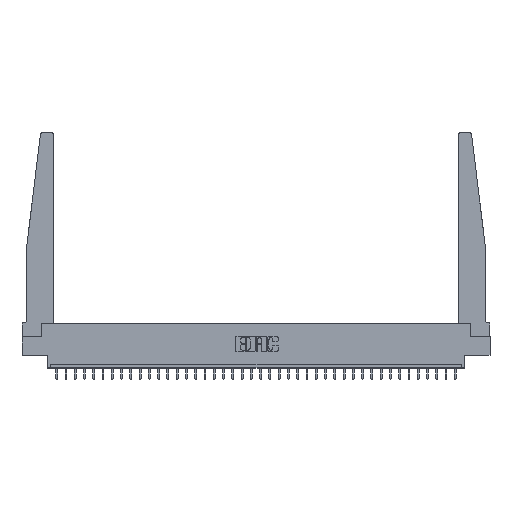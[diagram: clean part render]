
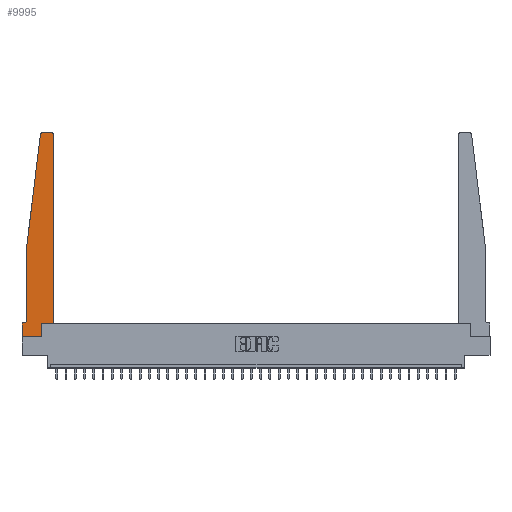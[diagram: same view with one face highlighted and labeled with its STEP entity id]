
A CAD part, top view. The second image highlights one B-rep face of the part: STEP entity #9995.
In plain terms, the highlighted planar face has unit normal (0, 0, 1).
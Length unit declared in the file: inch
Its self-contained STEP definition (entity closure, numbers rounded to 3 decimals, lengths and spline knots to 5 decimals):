
#300 = VERTEX_POINT ( 'NONE', #10481 ) ;
#734 = LINE ( 'NONE', #8101, #11076 ) ;
#1707 = DIRECTION ( 'NONE',  ( -0.122, -0.992, 0. ) ) ;
#1831 = FACE_OUTER_BOUND ( 'NONE', #9737, .T. ) ;
#2139 = EDGE_CURVE ( 'NONE', #7560, #2430, #734, .T. ) ;
#2144 = CARTESIAN_POINT ( 'NONE',  ( 0., 0., 0.37 ) ) ;
#2316 = CARTESIAN_POINT ( 'NONE',  ( 0.24675, 2.72367, 0.37 ) ) ;
#2386 = LINE ( 'NONE', #19761, #15559 ) ;
#2430 = VERTEX_POINT ( 'NONE', #7080 ) ;
#2535 = DIRECTION ( 'NONE',  ( 0., 0., -1. ) ) ;
#2603 = CARTESIAN_POINT ( 'NONE',  ( 0.425, 0.18, 0.37 ) ) ;
#2870 = DIRECTION ( 'NONE',  ( -1., 0., 0. ) ) ;
#3364 = DIRECTION ( 'NONE',  ( 0., -1., 0. ) ) ;
#3448 = AXIS2_PLACEMENT_3D ( 'NONE', #6725, #11809, #6570 ) ;
#3681 = EDGE_CURVE ( 'NONE', #2430, #6125, #12863, .T. ) ;
#4081 = CARTESIAN_POINT ( 'NONE',  ( 0.395, 2.75, 0.37 ) ) ;
#4702 = ORIENTED_EDGE ( 'NONE', *, *, #5469, .T. ) ;
#5469 = EDGE_CURVE ( 'NONE', #6577, #11866, #28727, .T. ) ;
#6125 = VERTEX_POINT ( 'NONE', #2316 ) ;
#6570 = DIRECTION ( 'NONE',  ( 1., 0., 0. ) ) ;
#6577 = VERTEX_POINT ( 'NONE', #20592 ) ;
#6643 = CARTESIAN_POINT ( 'NONE',  ( 0.2605, 0., 0.37 ) ) ;
#6725 = CARTESIAN_POINT ( 'NONE',  ( 0., 0.1875, 0.37 ) ) ;
#7080 = CARTESIAN_POINT ( 'NONE',  ( 0.27653, 2.75, 0.37 ) ) ;
#7560 = VERTEX_POINT ( 'NONE', #4081 ) ;
#7802 = EDGE_CURVE ( 'NONE', #300, #32115, #15045, .T. ) ;
#7805 = EDGE_CURVE ( 'NONE', #9225, #23556, #9787, .T. ) ;
#8101 = CARTESIAN_POINT ( 'NONE',  ( 0.25, 2.75, 0.37 ) ) ;
#9005 = DIRECTION ( 'NONE',  ( 1., 0., 0. ) ) ;
#9020 = CARTESIAN_POINT ( 'NONE',  ( 0., 0., 0.37 ) ) ;
#9225 = VERTEX_POINT ( 'NONE', #6643 ) ;
#9737 = EDGE_LOOP ( 'NONE', ( #20109, #15426, #15410, #4702, #16106, #26587, #24130, #14620, #29004, #9739, #24128, #9756 ) ) ;
#9739 = ORIENTED_EDGE ( 'NONE', *, *, #21697, .T. ) ;
#9756 = ORIENTED_EDGE ( 'NONE', *, *, #17944, .T. ) ;
#9787 = LINE ( 'NONE', #12593, #22171 ) ;
#9995 = ADVANCED_FACE ( 'NONE', ( #1831 ), #29013, .T. ) ;
#10481 = CARTESIAN_POINT ( 'NONE',  ( 0.425, 0.18, 0.37 ) ) ;
#10657 = DIRECTION ( 'NONE',  ( 1., 0., 0. ) ) ;
#10782 = LINE ( 'NONE', #21133, #31820 ) ;
#10863 = CARTESIAN_POINT ( 'NONE',  ( 0.065, 1.25, 0.37 ) ) ;
#10869 = AXIS2_PLACEMENT_3D ( 'NONE', #29723, #2535, #22856 ) ;
#11076 = VECTOR ( 'NONE', #2870, 39.37008 ) ;
#11333 = AXIS2_PLACEMENT_3D ( 'NONE', #21490, #31466, #9005 ) ;
#11809 = DIRECTION ( 'NONE',  ( 0., 0., 1. ) ) ;
#11866 = VERTEX_POINT ( 'NONE', #29800 ) ;
#12130 = DIRECTION ( 'NONE',  ( 0., -1., 0. ) ) ;
#12593 = CARTESIAN_POINT ( 'NONE',  ( 0.2605, 0.18, 0.37 ) ) ;
#12863 = CIRCLE ( 'NONE', #14942, 0.03 ) ;
#13383 = CARTESIAN_POINT ( 'NONE',  ( 0., 0., 0.37 ) ) ;
#14620 = ORIENTED_EDGE ( 'NONE', *, *, #26352, .T. ) ;
#14762 = VERTEX_POINT ( 'NONE', #32381 ) ;
#14942 = AXIS2_PLACEMENT_3D ( 'NONE', #15763, #18395, #10657 ) ;
#15045 = LINE ( 'NONE', #2603, #20067 ) ;
#15410 = ORIENTED_EDGE ( 'NONE', *, *, #22152, .T. ) ;
#15426 = ORIENTED_EDGE ( 'NONE', *, *, #3681, .T. ) ;
#15559 = VECTOR ( 'NONE', #16813, 39.37008 ) ;
#15763 = CARTESIAN_POINT ( 'NONE',  ( 0.27653, 2.72, 0.37 ) ) ;
#16106 = ORIENTED_EDGE ( 'NONE', *, *, #29680, .T. ) ;
#16571 = LINE ( 'NONE', #9020, #17307 ) ;
#16813 = DIRECTION ( 'NONE',  ( -1., 0., 0. ) ) ;
#17307 = VECTOR ( 'NONE', #24117, 39.37008 ) ;
#17919 = CARTESIAN_POINT ( 'NONE',  ( 0., 0.1875, 0.37 ) ) ;
#17944 = EDGE_CURVE ( 'NONE', #32115, #7560, #25486, .T. ) ;
#18082 = EDGE_CURVE ( 'NONE', #26295, #18791, #24584, .T. ) ;
#18395 = DIRECTION ( 'NONE',  ( 0., 0., 1. ) ) ;
#18791 = VERTEX_POINT ( 'NONE', #13383 ) ;
#18826 = DIRECTION ( 'NONE',  ( 1., 0., 0. ) ) ;
#19761 = CARTESIAN_POINT ( 'NONE',  ( 0.065, 0.1875, 0.37 ) ) ;
#20067 = VECTOR ( 'NONE', #32259, 39.37008 ) ;
#20109 = ORIENTED_EDGE ( 'NONE', *, *, #2139, .T. ) ;
#20200 = EDGE_CURVE ( 'NONE', #14762, #26295, #2386, .T. ) ;
#20592 = CARTESIAN_POINT ( 'NONE',  ( 0.065, 1.25, 0.37 ) ) ;
#21133 = CARTESIAN_POINT ( 'NONE',  ( 0.425, 0.18, 0.37 ) ) ;
#21490 = CARTESIAN_POINT ( 'NONE',  ( 0.395, 2.72, 0.37 ) ) ;
#21695 = CARTESIAN_POINT ( 'NONE',  ( 0.065, 1.25, 0.37 ) ) ;
#21697 = EDGE_CURVE ( 'NONE', #23556, #300, #10782, .T. ) ;
#21888 = CARTESIAN_POINT ( 'NONE',  ( 0.425, 2.72, 0.37 ) ) ;
#22152 = EDGE_CURVE ( 'NONE', #6125, #6577, #29214, .T. ) ;
#22171 = VECTOR ( 'NONE', #22602, 39.37008 ) ;
#22438 = VECTOR ( 'NONE', #1707, 39.37008 ) ;
#22602 = DIRECTION ( 'NONE',  ( 0., 1., 0. ) ) ;
#22856 = DIRECTION ( 'NONE',  ( -1., 0., 0. ) ) ;
#23556 = VERTEX_POINT ( 'NONE', #24685 ) ;
#24117 = DIRECTION ( 'NONE',  ( 1., 0., 0. ) ) ;
#24128 = ORIENTED_EDGE ( 'NONE', *, *, #7802, .T. ) ;
#24130 = ORIENTED_EDGE ( 'NONE', *, *, #18082, .T. ) ;
#24584 = LINE ( 'NONE', #2144, #29656 ) ;
#24685 = CARTESIAN_POINT ( 'NONE',  ( 0.2605, 0.18, 0.37 ) ) ;
#25486 = CIRCLE ( 'NONE', #11333, 0.03 ) ;
#25551 = CIRCLE ( 'NONE', #10869, 0.05 ) ;
#26295 = VERTEX_POINT ( 'NONE', #17919 ) ;
#26352 = EDGE_CURVE ( 'NONE', #18791, #9225, #16571, .T. ) ;
#26587 = ORIENTED_EDGE ( 'NONE', *, *, #20200, .T. ) ;
#28727 = LINE ( 'NONE', #10863, #29702 ) ;
#29004 = ORIENTED_EDGE ( 'NONE', *, *, #7805, .T. ) ;
#29013 = PLANE ( 'NONE',  #3448 ) ;
#29214 = LINE ( 'NONE', #21695, #22438 ) ;
#29656 = VECTOR ( 'NONE', #12130, 39.37008 ) ;
#29680 = EDGE_CURVE ( 'NONE', #11866, #14762, #25551, .T. ) ;
#29702 = VECTOR ( 'NONE', #3364, 39.37008 ) ;
#29723 = CARTESIAN_POINT ( 'NONE',  ( 0.015, 0.2375, 0.37 ) ) ;
#29800 = CARTESIAN_POINT ( 'NONE',  ( 0.065, 0.2375, 0.37 ) ) ;
#31466 = DIRECTION ( 'NONE',  ( 0., 0., 1. ) ) ;
#31820 = VECTOR ( 'NONE', #18826, 39.37008 ) ;
#32115 = VERTEX_POINT ( 'NONE', #21888 ) ;
#32259 = DIRECTION ( 'NONE',  ( 0., 1., 0. ) ) ;
#32381 = CARTESIAN_POINT ( 'NONE',  ( 0.015, 0.1875, 0.37 ) ) ;
